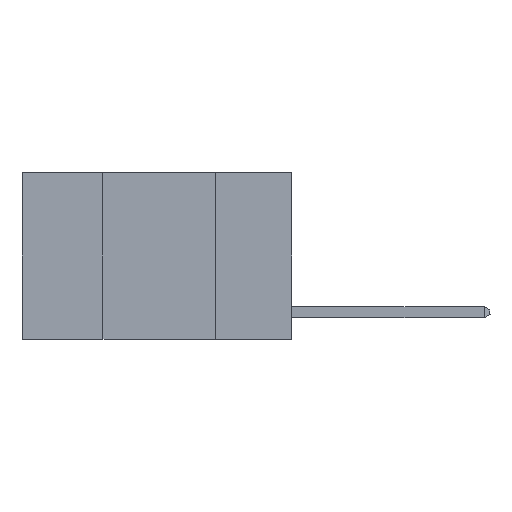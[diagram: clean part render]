
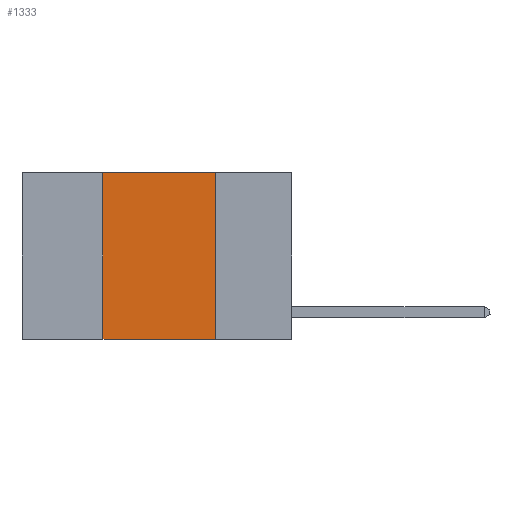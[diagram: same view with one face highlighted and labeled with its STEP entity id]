
A CAD part, left-side view. The second image highlights one B-rep face of the part: STEP entity #1333.
In plain terms, the highlighted planar face has unit normal (-1, 0, 0).
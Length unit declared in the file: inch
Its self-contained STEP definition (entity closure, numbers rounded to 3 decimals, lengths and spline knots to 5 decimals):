
#579 = VERTEX_POINT ( 'NONE', #4680 ) ;
#1329 = DIRECTION ( 'NONE',  ( 0., 0., 1. ) ) ;
#1333 = ADVANCED_FACE ( 'NONE', ( #8880 ), #9875, .F. ) ;
#1544 = AXIS2_PLACEMENT_3D ( 'NONE', #3507, #9758, #5336 ) ;
#1608 = VECTOR ( 'NONE', #1329, 39.37008 ) ;
#1656 = ORIENTED_EDGE ( 'NONE', *, *, #7166, .F. ) ;
#1955 = EDGE_CURVE ( 'NONE', #4111, #11280, #6463, .T. ) ;
#3249 = EDGE_LOOP ( 'NONE', ( #3463, #11397, #1656, #11375 ) ) ;
#3463 = ORIENTED_EDGE ( 'NONE', *, *, #10555, .F. ) ;
#3507 = CARTESIAN_POINT ( 'NONE',  ( 0., 0.6, 0. ) ) ;
#3677 = VECTOR ( 'NONE', #10072, 39.37008 ) ;
#3708 = VECTOR ( 'NONE', #7391, 39.37008 ) ;
#4111 = VERTEX_POINT ( 'NONE', #8216 ) ;
#4680 = CARTESIAN_POINT ( 'NONE',  ( 0., 0.42, -0.37 ) ) ;
#4789 = CARTESIAN_POINT ( 'NONE',  ( 0., 0.17, -0.37 ) ) ;
#4858 = VERTEX_POINT ( 'NONE', #4789 ) ;
#5336 = DIRECTION ( 'NONE',  ( 0., 0., -1. ) ) ;
#5895 = VECTOR ( 'NONE', #8572, 39.37008 ) ;
#6463 = LINE ( 'NONE', #10185, #3677 ) ;
#6653 = LINE ( 'NONE', #10262, #5895 ) ;
#7166 = EDGE_CURVE ( 'NONE', #579, #4111, #10641, .T. ) ;
#7391 = DIRECTION ( 'NONE',  ( 0., -1., 0. ) ) ;
#8216 = CARTESIAN_POINT ( 'NONE',  ( 0., 0.42, 0. ) ) ;
#8287 = CARTESIAN_POINT ( 'NONE',  ( 0., 0.6, -0.37 ) ) ;
#8572 = DIRECTION ( 'NONE',  ( 0., 0., -1. ) ) ;
#8880 = FACE_OUTER_BOUND ( 'NONE', #3249, .T. ) ;
#9338 = CARTESIAN_POINT ( 'NONE',  ( 0., 0.42, 0. ) ) ;
#9470 = EDGE_CURVE ( 'NONE', #579, #4858, #11051, .T. ) ;
#9758 = DIRECTION ( 'NONE',  ( 1., 0., 0. ) ) ;
#9875 = PLANE ( 'NONE',  #1544 ) ;
#10072 = DIRECTION ( 'NONE',  ( 0., -1., 0. ) ) ;
#10185 = CARTESIAN_POINT ( 'NONE',  ( 0., 0.6, 0. ) ) ;
#10262 = CARTESIAN_POINT ( 'NONE',  ( 0., 0.17, 0. ) ) ;
#10449 = CARTESIAN_POINT ( 'NONE',  ( 0., 0.17, 0. ) ) ;
#10555 = EDGE_CURVE ( 'NONE', #11280, #4858, #6653, .T. ) ;
#10641 = LINE ( 'NONE', #9338, #1608 ) ;
#11051 = LINE ( 'NONE', #8287, #3708 ) ;
#11280 = VERTEX_POINT ( 'NONE', #10449 ) ;
#11375 = ORIENTED_EDGE ( 'NONE', *, *, #9470, .T. ) ;
#11397 = ORIENTED_EDGE ( 'NONE', *, *, #1955, .F. ) ;
